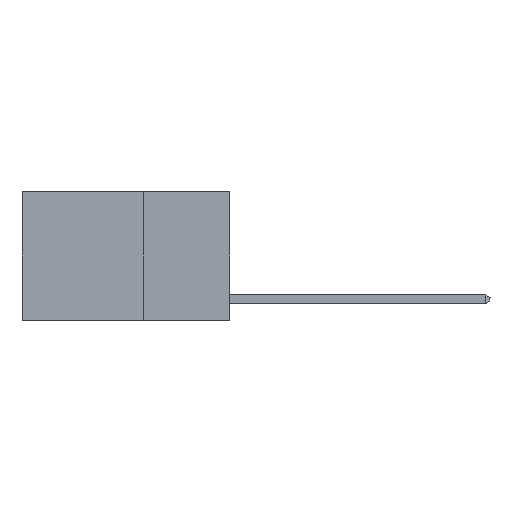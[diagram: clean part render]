
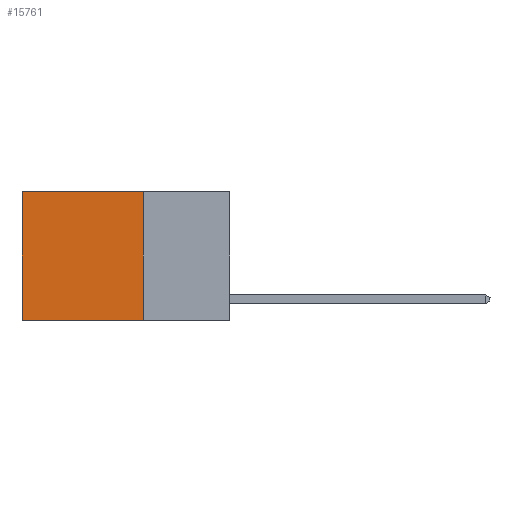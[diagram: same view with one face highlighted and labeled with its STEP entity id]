
A CAD part, left-side view. The second image highlights one B-rep face of the part: STEP entity #15761.
In plain terms, the highlighted planar face has unit normal (-1, 0, 0).
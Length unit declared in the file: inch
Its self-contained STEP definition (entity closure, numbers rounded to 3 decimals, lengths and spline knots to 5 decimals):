
#147 = FACE_OUTER_BOUND ( 'NONE', #18513, .T. ) ;
#442 = AXIS2_PLACEMENT_3D ( 'NONE', #3735, #14113, #5030 ) ;
#2132 = LINE ( 'NONE', #7816, #21202 ) ;
#2593 = DIRECTION ( 'NONE',  ( 0., 0., -1. ) ) ;
#3241 = CARTESIAN_POINT ( 'NONE',  ( 0.2625, 0.6, 0. ) ) ;
#3735 = CARTESIAN_POINT ( 'NONE',  ( 0.2625, 0.25, 0. ) ) ;
#4328 = VERTEX_POINT ( 'NONE', #9523 ) ;
#5030 = DIRECTION ( 'NONE',  ( 0., 0., -1. ) ) ;
#6350 = DIRECTION ( 'NONE',  ( 0., 1., 0. ) ) ;
#7816 = CARTESIAN_POINT ( 'NONE',  ( 0.2625, 0.25, 0. ) ) ;
#8061 = CARTESIAN_POINT ( 'NONE',  ( 0.2625, 0.25, -0.37 ) ) ;
#9523 = CARTESIAN_POINT ( 'NONE',  ( 0.2625, 0.6, 0. ) ) ;
#9706 = EDGE_CURVE ( 'NONE', #18411, #4328, #21107, .T. ) ;
#9820 = DIRECTION ( 'NONE',  ( 0., 1., 0. ) ) ;
#9929 = CARTESIAN_POINT ( 'NONE',  ( 0.2625, 0.25, -0.37 ) ) ;
#10576 = EDGE_CURVE ( 'NONE', #21065, #11329, #22647, .T. ) ;
#10749 = PLANE ( 'NONE',  #442 ) ;
#10827 = VECTOR ( 'NONE', #16121, 39.37008 ) ;
#11329 = VERTEX_POINT ( 'NONE', #19063 ) ;
#12891 = VECTOR ( 'NONE', #9820, 39.37008 ) ;
#13776 = ORIENTED_EDGE ( 'NONE', *, *, #20900, .T. ) ;
#14113 = DIRECTION ( 'NONE',  ( 1., 0., 0. ) ) ;
#14190 = ORIENTED_EDGE ( 'NONE', *, *, #20294, .F. ) ;
#15160 = ORIENTED_EDGE ( 'NONE', *, *, #9706, .T. ) ;
#15761 = ADVANCED_FACE ( 'NONE', ( #147 ), #10749, .F. ) ;
#16121 = DIRECTION ( 'NONE',  ( 0., 0., -1. ) ) ;
#18282 = CARTESIAN_POINT ( 'NONE',  ( 0.2625, 0.25, 0. ) ) ;
#18411 = VERTEX_POINT ( 'NONE', #18282 ) ;
#18513 = EDGE_LOOP ( 'NONE', ( #13776, #19309, #14190, #15160 ) ) ;
#19063 = CARTESIAN_POINT ( 'NONE',  ( 0.2625, 0.6, -0.37 ) ) ;
#19309 = ORIENTED_EDGE ( 'NONE', *, *, #10576, .F. ) ;
#19616 = LINE ( 'NONE', #3241, #10827 ) ;
#20294 = EDGE_CURVE ( 'NONE', #18411, #21065, #2132, .T. ) ;
#20900 = EDGE_CURVE ( 'NONE', #4328, #11329, #19616, .T. ) ;
#21065 = VERTEX_POINT ( 'NONE', #8061 ) ;
#21107 = LINE ( 'NONE', #22648, #12891 ) ;
#21202 = VECTOR ( 'NONE', #2593, 39.37008 ) ;
#22647 = LINE ( 'NONE', #9929, #22781 ) ;
#22648 = CARTESIAN_POINT ( 'NONE',  ( 0.2625, 0.25, 0. ) ) ;
#22781 = VECTOR ( 'NONE', #6350, 39.37008 ) ;
